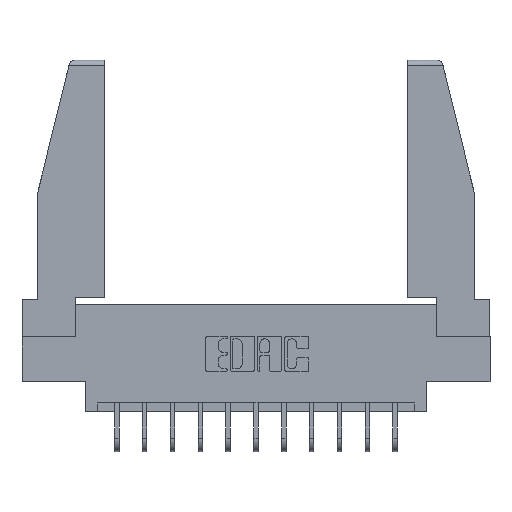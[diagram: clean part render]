
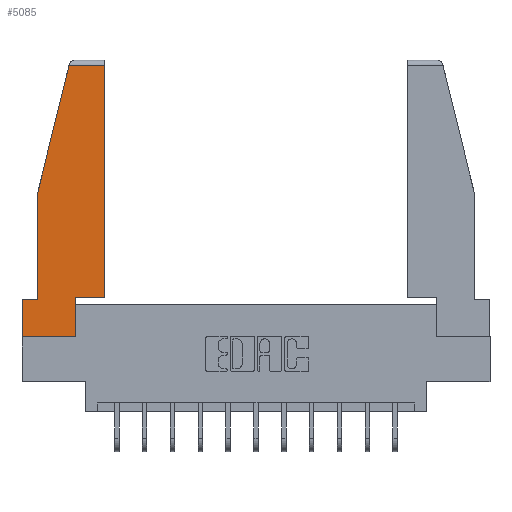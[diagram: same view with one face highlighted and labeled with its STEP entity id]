
A CAD part, top view. The second image highlights one B-rep face of the part: STEP entity #5085.
In plain terms, the highlighted planar face has unit normal (0, 0, 1).
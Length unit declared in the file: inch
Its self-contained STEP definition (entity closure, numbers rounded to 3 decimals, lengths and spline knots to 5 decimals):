
#63 = PLANE ( 'NONE',  #15180 ) ;
#472 = VERTEX_POINT ( 'NONE', #11945 ) ;
#644 = ORIENTED_EDGE ( 'NONE', *, *, #7437, .T. ) ;
#649 = CARTESIAN_POINT ( 'NONE',  ( 0.086, 0.8, 0. ) ) ;
#686 = CARTESIAN_POINT ( 'NONE',  ( 0., 0., 0. ) ) ;
#1258 = ORIENTED_EDGE ( 'NONE', *, *, #14563, .T. ) ;
#1464 = CARTESIAN_POINT ( 'NONE',  ( 0., 0.21, 0. ) ) ;
#1493 = CARTESIAN_POINT ( 'NONE',  ( 0., 0., 0. ) ) ;
#1574 = CARTESIAN_POINT ( 'NONE',  ( 0., 0.21, 0. ) ) ;
#1790 = CARTESIAN_POINT ( 'NONE',  ( 0.461, 0.223, 0. ) ) ;
#2629 = VECTOR ( 'NONE', #12639, 39.37008 ) ;
#2738 = LINE ( 'NONE', #11557, #15795 ) ;
#3092 = CARTESIAN_POINT ( 'NONE',  ( 0.461, 0.223, 0. ) ) ;
#3191 = EDGE_CURVE ( 'NONE', #12447, #5401, #11829, .T. ) ;
#3819 = LINE ( 'NONE', #12711, #12587 ) ;
#3879 = ORIENTED_EDGE ( 'NONE', *, *, #10964, .T. ) ;
#4000 = VECTOR ( 'NONE', #14553, 39.37008 ) ;
#4306 = VERTEX_POINT ( 'NONE', #9697 ) ;
#4331 = VERTEX_POINT ( 'NONE', #686 ) ;
#4599 = LINE ( 'NONE', #10617, #13366 ) ;
#4607 = ORIENTED_EDGE ( 'NONE', *, *, #11934, .T. ) ;
#4836 = DIRECTION ( 'NONE',  ( 0., 1., 0. ) ) ;
#4901 = VECTOR ( 'NONE', #8516, 39.37008 ) ;
#5034 = CARTESIAN_POINT ( 'NONE',  ( 0.297, 0., 0. ) ) ;
#5085 = ADVANCED_FACE ( 'NONE', ( #9114 ), #63, .T. ) ;
#5401 = VERTEX_POINT ( 'NONE', #3092 ) ;
#5926 = LINE ( 'NONE', #12624, #6142 ) ;
#6102 = DIRECTION ( 'NONE',  ( -1., 0., 0. ) ) ;
#6142 = VECTOR ( 'NONE', #6102, 39.37008 ) ;
#6388 = VECTOR ( 'NONE', #14734, 39.37008 ) ;
#7189 = CARTESIAN_POINT ( 'NONE',  ( 0.297, 0.223, 0. ) ) ;
#7284 = VERTEX_POINT ( 'NONE', #649 ) ;
#7437 = EDGE_CURVE ( 'NONE', #4306, #10000, #5926, .T. ) ;
#7927 = EDGE_LOOP ( 'NONE', ( #4607, #14557, #3879, #12691, #644, #1258, #13662, #11599, #15871 ) ) ;
#8293 = LINE ( 'NONE', #1464, #13006 ) ;
#8516 = DIRECTION ( 'NONE',  ( 1., 0., 0. ) ) ;
#9114 = FACE_OUTER_BOUND ( 'NONE', #7927, .T. ) ;
#9697 = CARTESIAN_POINT ( 'NONE',  ( 0.086, 0.21, 0. ) ) ;
#10000 = VERTEX_POINT ( 'NONE', #1574 ) ;
#10137 = DIRECTION ( 'NONE',  ( -1., 0., 0. ) ) ;
#10165 = DIRECTION ( 'NONE',  ( 0., -1., 0. ) ) ;
#10418 = DIRECTION ( 'NONE',  ( 0., -1., 0. ) ) ;
#10471 = LINE ( 'NONE', #13233, #4000 ) ;
#10506 = DIRECTION ( 'NONE',  ( 1., 0., 0. ) ) ;
#10617 = CARTESIAN_POINT ( 'NONE',  ( 0., 1.52, 0. ) ) ;
#10964 = EDGE_CURVE ( 'NONE', #16161, #7284, #10471, .T. ) ;
#10990 = EDGE_CURVE ( 'NONE', #472, #16161, #4599, .T. ) ;
#11557 = CARTESIAN_POINT ( 'NONE',  ( 0.086, 0.8, 0. ) ) ;
#11599 = ORIENTED_EDGE ( 'NONE', *, *, #14910, .T. ) ;
#11829 = LINE ( 'NONE', #7189, #4901 ) ;
#11934 = EDGE_CURVE ( 'NONE', #5401, #472, #15815, .T. ) ;
#11945 = CARTESIAN_POINT ( 'NONE',  ( 0.461, 1.52, 0. ) ) ;
#12416 = EDGE_CURVE ( 'NONE', #7284, #4306, #2738, .T. ) ;
#12447 = VERTEX_POINT ( 'NONE', #13572 ) ;
#12587 = VECTOR ( 'NONE', #4836, 39.37008 ) ;
#12624 = CARTESIAN_POINT ( 'NONE',  ( 0., 0.21, 0. ) ) ;
#12639 = DIRECTION ( 'NONE',  ( 1., 0., 0. ) ) ;
#12691 = ORIENTED_EDGE ( 'NONE', *, *, #12416, .T. ) ;
#12711 = CARTESIAN_POINT ( 'NONE',  ( 0.297, 0., 0. ) ) ;
#13006 = VECTOR ( 'NONE', #10418, 39.37008 ) ;
#13233 = CARTESIAN_POINT ( 'NONE',  ( 0.271, 1.55, 0. ) ) ;
#13366 = VECTOR ( 'NONE', #10137, 39.37008 ) ;
#13572 = CARTESIAN_POINT ( 'NONE',  ( 0.297, 0.223, 0. ) ) ;
#13662 = ORIENTED_EDGE ( 'NONE', *, *, #14390, .T. ) ;
#14390 = EDGE_CURVE ( 'NONE', #4331, #14461, #16092, .T. ) ;
#14461 = VERTEX_POINT ( 'NONE', #5034 ) ;
#14480 = CARTESIAN_POINT ( 'NONE',  ( 0.2636, 1.52, 0. ) ) ;
#14552 = DIRECTION ( 'NONE',  ( 0., 0., 1. ) ) ;
#14553 = DIRECTION ( 'NONE',  ( -0.239, -0.971, 0. ) ) ;
#14557 = ORIENTED_EDGE ( 'NONE', *, *, #10990, .T. ) ;
#14563 = EDGE_CURVE ( 'NONE', #10000, #4331, #8293, .T. ) ;
#14734 = DIRECTION ( 'NONE',  ( 0., 1., 0. ) ) ;
#14910 = EDGE_CURVE ( 'NONE', #14461, #12447, #3819, .T. ) ;
#15180 = AXIS2_PLACEMENT_3D ( 'NONE', #1493, #14552, #10506 ) ;
#15795 = VECTOR ( 'NONE', #10165, 39.37008 ) ;
#15815 = LINE ( 'NONE', #1790, #6388 ) ;
#15871 = ORIENTED_EDGE ( 'NONE', *, *, #3191, .T. ) ;
#16092 = LINE ( 'NONE', #16728, #2629 ) ;
#16161 = VERTEX_POINT ( 'NONE', #14480 ) ;
#16728 = CARTESIAN_POINT ( 'NONE',  ( 0., 0., 0. ) ) ;
